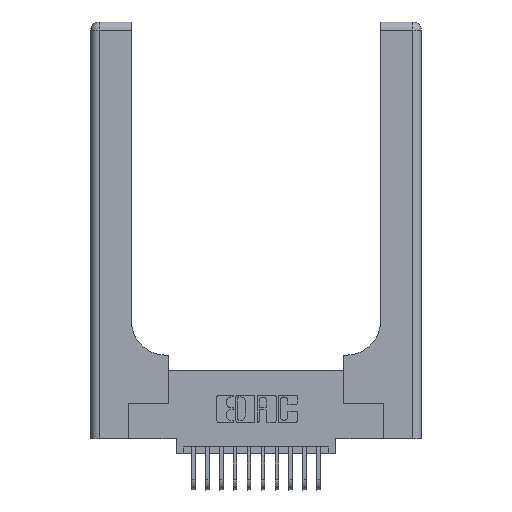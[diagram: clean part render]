
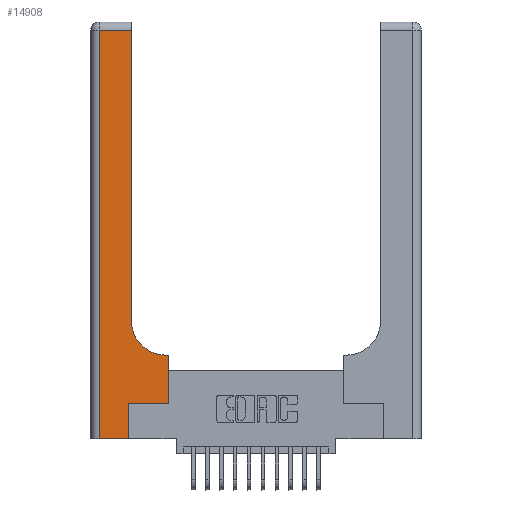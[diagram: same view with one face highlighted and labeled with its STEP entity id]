
A CAD part, top view. The second image highlights one B-rep face of the part: STEP entity #14908.
In plain terms, the highlighted planar face has unit normal (0, 0, 1).
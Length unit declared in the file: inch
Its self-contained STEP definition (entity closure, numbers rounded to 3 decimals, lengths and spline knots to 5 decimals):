
#54 = LINE ( 'NONE', #6651, #10625 ) ;
#131 = LINE ( 'NONE', #1691, #12540 ) ;
#268 = EDGE_CURVE ( 'NONE', #12240, #1881, #8241, .T. ) ;
#528 = ORIENTED_EDGE ( 'NONE', *, *, #18549, .T. ) ;
#696 = PLANE ( 'NONE',  #15950 ) ;
#1188 = FACE_OUTER_BOUND ( 'NONE', #17496, .T. ) ;
#1313 = CARTESIAN_POINT ( 'NONE',  ( 0.06, 3., 0.37 ) ) ;
#1390 = CARTESIAN_POINT ( 'NONE',  ( 0.06, 2.94, 0.37 ) ) ;
#1536 = CARTESIAN_POINT ( 'NONE',  ( 0.5415, 0.6, 0.37 ) ) ;
#1608 = ORIENTED_EDGE ( 'NONE', *, *, #15918, .T. ) ;
#1691 = CARTESIAN_POINT ( 'NONE',  ( 0.2915, 0.6, 0.37 ) ) ;
#1861 = ORIENTED_EDGE ( 'NONE', *, *, #3249, .T. ) ;
#1881 = VERTEX_POINT ( 'NONE', #10887 ) ;
#2279 = VECTOR ( 'NONE', #11718, 39.37008 ) ;
#2303 = CARTESIAN_POINT ( 'NONE',  ( 0., 3., 0.37 ) ) ;
#2673 = VERTEX_POINT ( 'NONE', #15232 ) ;
#3008 = EDGE_CURVE ( 'NONE', #12258, #2673, #18155, .T. ) ;
#3051 = CARTESIAN_POINT ( 'NONE',  ( 0.5585, 0.6, 0.37 ) ) ;
#3249 = EDGE_CURVE ( 'NONE', #2673, #7933, #17020, .T. ) ;
#3635 = DIRECTION ( 'NONE',  ( 1., 0., 0. ) ) ;
#3935 = DIRECTION ( 'NONE',  ( 0., 0., -1. ) ) ;
#4299 = VERTEX_POINT ( 'NONE', #17787 ) ;
#5674 = CARTESIAN_POINT ( 'NONE',  ( 0.5585, 0.25, 0.37 ) ) ;
#5719 = VERTEX_POINT ( 'NONE', #7976 ) ;
#5773 = ORIENTED_EDGE ( 'NONE', *, *, #268, .T. ) ;
#6651 = CARTESIAN_POINT ( 'NONE',  ( 0., 2.94, 0.37 ) ) ;
#7154 = VECTOR ( 'NONE', #14093, 39.37008 ) ;
#7283 = LINE ( 'NONE', #12974, #15029 ) ;
#7602 = LINE ( 'NONE', #12648, #7154 ) ;
#7933 = VERTEX_POINT ( 'NONE', #15835 ) ;
#7976 = CARTESIAN_POINT ( 'NONE',  ( 0.269, 0., 0.37 ) ) ;
#7990 = EDGE_CURVE ( 'NONE', #14710, #4299, #17834, .T. ) ;
#8200 = DIRECTION ( 'NONE',  ( 0., 0., -1. ) ) ;
#8241 = LINE ( 'NONE', #16039, #11677 ) ;
#8613 = VERTEX_POINT ( 'NONE', #3051 ) ;
#8777 = ORIENTED_EDGE ( 'NONE', *, *, #8854, .T. ) ;
#8854 = EDGE_CURVE ( 'NONE', #5719, #12240, #7602, .T. ) ;
#9769 = VECTOR ( 'NONE', #14700, 39.37008 ) ;
#10585 = DIRECTION ( 'NONE',  ( -1., 0., 0. ) ) ;
#10625 = VECTOR ( 'NONE', #12505, 39.37008 ) ;
#10887 = CARTESIAN_POINT ( 'NONE',  ( 0.5585, 0.25, 0.37 ) ) ;
#11271 = VECTOR ( 'NONE', #15876, 39.37008 ) ;
#11677 = VECTOR ( 'NONE', #3635, 39.37008 ) ;
#11718 = DIRECTION ( 'NONE',  ( 0., -1., 0. ) ) ;
#11897 = EDGE_CURVE ( 'NONE', #7933, #14710, #54, .T. ) ;
#12240 = VERTEX_POINT ( 'NONE', #13304 ) ;
#12258 = VERTEX_POINT ( 'NONE', #1536 ) ;
#12445 = ORIENTED_EDGE ( 'NONE', *, *, #13115, .T. ) ;
#12505 = DIRECTION ( 'NONE',  ( -1., 0., 0. ) ) ;
#12540 = VECTOR ( 'NONE', #10585, 39.37008 ) ;
#12648 = CARTESIAN_POINT ( 'NONE',  ( 0.269, 0., 0.37 ) ) ;
#12741 = CARTESIAN_POINT ( 'NONE',  ( 0.5415, 0.85, 0.37 ) ) ;
#12974 = CARTESIAN_POINT ( 'NONE',  ( 0., 0., 0.37 ) ) ;
#13115 = EDGE_CURVE ( 'NONE', #1881, #8613, #14687, .T. ) ;
#13290 = CARTESIAN_POINT ( 'NONE',  ( 0.2915, 3., 0.37 ) ) ;
#13304 = CARTESIAN_POINT ( 'NONE',  ( 0.269, 0.25, 0.37 ) ) ;
#14070 = DIRECTION ( 'NONE',  ( -1., 0., 0. ) ) ;
#14093 = DIRECTION ( 'NONE',  ( 0., 1., 0. ) ) ;
#14202 = DIRECTION ( 'NONE',  ( 1., 0., 0. ) ) ;
#14449 = DIRECTION ( 'NONE',  ( 1., 0., 0. ) ) ;
#14687 = LINE ( 'NONE', #5674, #11271 ) ;
#14700 = DIRECTION ( 'NONE',  ( 0., 1., 0. ) ) ;
#14710 = VERTEX_POINT ( 'NONE', #1390 ) ;
#14908 = ADVANCED_FACE ( 'NONE', ( #1188 ), #696, .F. ) ;
#15029 = VECTOR ( 'NONE', #14449, 39.37008 ) ;
#15232 = CARTESIAN_POINT ( 'NONE',  ( 0.2915, 0.85, 0.37 ) ) ;
#15803 = ORIENTED_EDGE ( 'NONE', *, *, #7990, .T. ) ;
#15835 = CARTESIAN_POINT ( 'NONE',  ( 0.2915, 2.94, 0.37 ) ) ;
#15876 = DIRECTION ( 'NONE',  ( 0., 1., 0. ) ) ;
#15918 = EDGE_CURVE ( 'NONE', #8613, #12258, #131, .T. ) ;
#15950 = AXIS2_PLACEMENT_3D ( 'NONE', #2303, #8200, #14070 ) ;
#16039 = CARTESIAN_POINT ( 'NONE',  ( 0.269, 0.25, 0.37 ) ) ;
#16059 = AXIS2_PLACEMENT_3D ( 'NONE', #12741, #3935, #14202 ) ;
#16211 = ORIENTED_EDGE ( 'NONE', *, *, #11897, .T. ) ;
#17020 = LINE ( 'NONE', #13290, #9769 ) ;
#17496 = EDGE_LOOP ( 'NONE', ( #1861, #16211, #15803, #528, #8777, #5773, #12445, #1608, #17660 ) ) ;
#17660 = ORIENTED_EDGE ( 'NONE', *, *, #3008, .T. ) ;
#17787 = CARTESIAN_POINT ( 'NONE',  ( 0.06, 0., 0.37 ) ) ;
#17834 = LINE ( 'NONE', #1313, #2279 ) ;
#18155 = CIRCLE ( 'NONE', #16059, 0.25 ) ;
#18549 = EDGE_CURVE ( 'NONE', #4299, #5719, #7283, .T. ) ;
